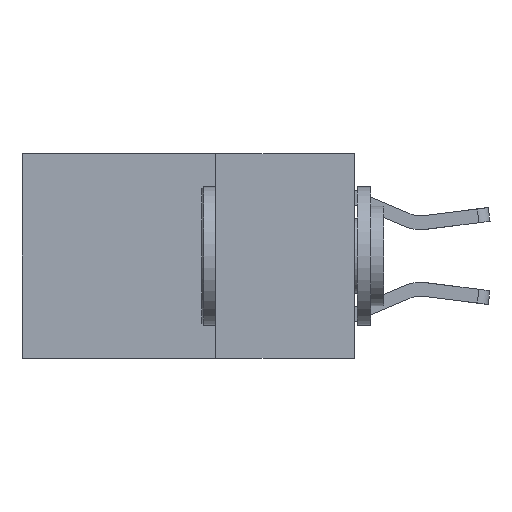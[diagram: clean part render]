
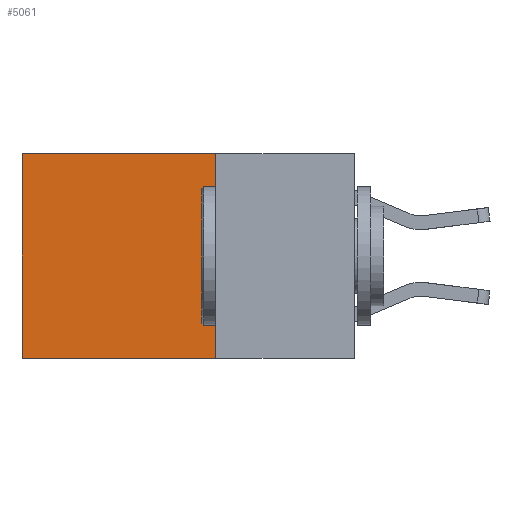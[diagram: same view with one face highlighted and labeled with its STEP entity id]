
A CAD part, left-side view. The second image highlights one B-rep face of the part: STEP entity #5061.
In plain terms, the highlighted planar face has unit normal (-1, 0, 0).
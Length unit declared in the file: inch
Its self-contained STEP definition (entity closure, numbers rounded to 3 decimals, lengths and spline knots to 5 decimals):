
#71 = LINE ( 'NONE', #898, #2185 ) ;
#137 = CARTESIAN_POINT ( 'NONE',  ( 0.2625, 0.25, 0. ) ) ;
#530 = CARTESIAN_POINT ( 'NONE',  ( 0.2625, 0.6, 0. ) ) ;
#898 = CARTESIAN_POINT ( 'NONE',  ( 0.2625, 0.25, -0.37 ) ) ;
#1005 = DIRECTION ( 'NONE',  ( 0., 1., 0. ) ) ;
#1232 = EDGE_LOOP ( 'NONE', ( #9164, #2935, #7996, #4695 ) ) ;
#1597 = CARTESIAN_POINT ( 'NONE',  ( 0.2625, 0.25, 0. ) ) ;
#1609 = LINE ( 'NONE', #9025, #4835 ) ;
#2185 = VECTOR ( 'NONE', #1005, 39.37008 ) ;
#2935 = ORIENTED_EDGE ( 'NONE', *, *, #8064, .F. ) ;
#3291 = VECTOR ( 'NONE', #8748, 39.37008 ) ;
#3842 = VERTEX_POINT ( 'NONE', #7695 ) ;
#4042 = CARTESIAN_POINT ( 'NONE',  ( 0.2625, 0.25, -0.37 ) ) ;
#4168 = VERTEX_POINT ( 'NONE', #7072 ) ;
#4472 = EDGE_CURVE ( 'NONE', #3842, #8234, #1609, .T. ) ;
#4485 = VERTEX_POINT ( 'NONE', #7401 ) ;
#4596 = DIRECTION ( 'NONE',  ( 1., 0., 0. ) ) ;
#4695 = ORIENTED_EDGE ( 'NONE', *, *, #8664, .T. ) ;
#4835 = VECTOR ( 'NONE', #6678, 39.37008 ) ;
#4923 = LINE ( 'NONE', #530, #3291 ) ;
#5061 = ADVANCED_FACE ( 'NONE', ( #5322 ), #8281, .F. ) ;
#5322 = FACE_OUTER_BOUND ( 'NONE', #1232, .T. ) ;
#5430 = DIRECTION ( 'NONE',  ( 0., 1., 0. ) ) ;
#6678 = DIRECTION ( 'NONE',  ( 0., 0., -1. ) ) ;
#6801 = DIRECTION ( 'NONE',  ( 0., 0., -1. ) ) ;
#7035 = EDGE_CURVE ( 'NONE', #4168, #4485, #4923, .T. ) ;
#7072 = CARTESIAN_POINT ( 'NONE',  ( 0.2625, 0.6, 0. ) ) ;
#7148 = AXIS2_PLACEMENT_3D ( 'NONE', #1597, #4596, #6801 ) ;
#7310 = LINE ( 'NONE', #137, #7334 ) ;
#7334 = VECTOR ( 'NONE', #5430, 39.37008 ) ;
#7401 = CARTESIAN_POINT ( 'NONE',  ( 0.2625, 0.6, -0.37 ) ) ;
#7695 = CARTESIAN_POINT ( 'NONE',  ( 0.2625, 0.25, 0. ) ) ;
#7996 = ORIENTED_EDGE ( 'NONE', *, *, #4472, .F. ) ;
#8064 = EDGE_CURVE ( 'NONE', #8234, #4485, #71, .T. ) ;
#8234 = VERTEX_POINT ( 'NONE', #4042 ) ;
#8281 = PLANE ( 'NONE',  #7148 ) ;
#8664 = EDGE_CURVE ( 'NONE', #3842, #4168, #7310, .T. ) ;
#8748 = DIRECTION ( 'NONE',  ( 0., 0., -1. ) ) ;
#9025 = CARTESIAN_POINT ( 'NONE',  ( 0.2625, 0.25, 0. ) ) ;
#9164 = ORIENTED_EDGE ( 'NONE', *, *, #7035, .T. ) ;
